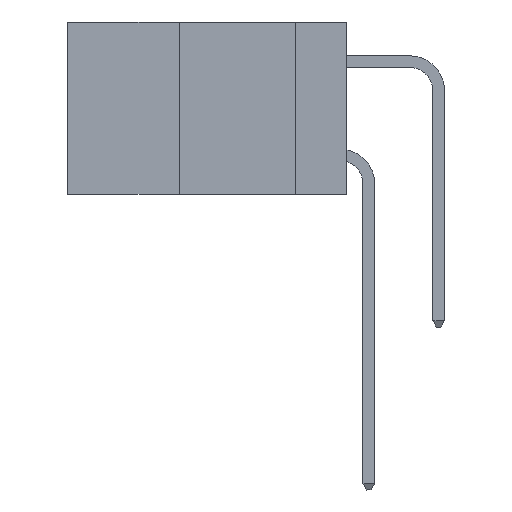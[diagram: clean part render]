
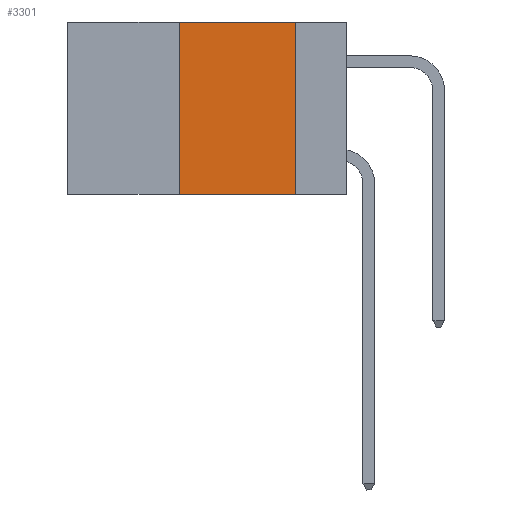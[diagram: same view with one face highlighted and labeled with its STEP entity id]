
A CAD part, left-side view. The second image highlights one B-rep face of the part: STEP entity #3301.
In plain terms, the highlighted planar face has unit normal (-1, 0, 0).
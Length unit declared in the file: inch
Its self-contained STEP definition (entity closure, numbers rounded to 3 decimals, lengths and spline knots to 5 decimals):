
#32 = LINE ( 'NONE', #3934, #11040 ) ;
#1333 = CARTESIAN_POINT ( 'NONE',  ( 0., 0.6, 0. ) ) ;
#1465 = ORIENTED_EDGE ( 'NONE', *, *, #13964, .T. ) ;
#2509 = DIRECTION ( 'NONE',  ( 0., -1., 0. ) ) ;
#3301 = ADVANCED_FACE ( 'NONE', ( #13398 ), #12016, .F. ) ;
#3934 = CARTESIAN_POINT ( 'NONE',  ( 0., 0.36, 0. ) ) ;
#3945 = DIRECTION ( 'NONE',  ( 0., 0., -1. ) ) ;
#3978 = DIRECTION ( 'NONE',  ( 1., 0., 0. ) ) ;
#4523 = EDGE_LOOP ( 'NONE', ( #9824, #4733, #11554, #1465 ) ) ;
#4532 = VECTOR ( 'NONE', #5511, 39.37008 ) ;
#4733 = ORIENTED_EDGE ( 'NONE', *, *, #16162, .F. ) ;
#5443 = CARTESIAN_POINT ( 'NONE',  ( 0., 0.11, 0. ) ) ;
#5511 = DIRECTION ( 'NONE',  ( 0., -1., 0. ) ) ;
#5872 = VERTEX_POINT ( 'NONE', #7890 ) ;
#6411 = LINE ( 'NONE', #7959, #9127 ) ;
#7386 = CARTESIAN_POINT ( 'NONE',  ( 0., 0.36, 0. ) ) ;
#7890 = CARTESIAN_POINT ( 'NONE',  ( 0., 0.11, -0.37 ) ) ;
#7959 = CARTESIAN_POINT ( 'NONE',  ( 0., 0.11, 0. ) ) ;
#7994 = CARTESIAN_POINT ( 'NONE',  ( 0., 0.6, 0. ) ) ;
#8375 = LINE ( 'NONE', #9251, #11103 ) ;
#8546 = CARTESIAN_POINT ( 'NONE',  ( 0., 0.36, -0.37 ) ) ;
#8798 = VERTEX_POINT ( 'NONE', #5443 ) ;
#9127 = VECTOR ( 'NONE', #3945, 39.37008 ) ;
#9251 = CARTESIAN_POINT ( 'NONE',  ( 0., 0.6, -0.37 ) ) ;
#9824 = ORIENTED_EDGE ( 'NONE', *, *, #16711, .F. ) ;
#9827 = VERTEX_POINT ( 'NONE', #8546 ) ;
#11040 = VECTOR ( 'NONE', #14700, 39.37008 ) ;
#11103 = VECTOR ( 'NONE', #2509, 39.37008 ) ;
#11554 = ORIENTED_EDGE ( 'NONE', *, *, #12784, .F. ) ;
#12016 = PLANE ( 'NONE',  #13659 ) ;
#12784 = EDGE_CURVE ( 'NONE', #9827, #15742, #32, .T. ) ;
#13398 = FACE_OUTER_BOUND ( 'NONE', #4523, .T. ) ;
#13431 = DIRECTION ( 'NONE',  ( 0., 0., -1. ) ) ;
#13659 = AXIS2_PLACEMENT_3D ( 'NONE', #7994, #3978, #13431 ) ;
#13964 = EDGE_CURVE ( 'NONE', #9827, #5872, #8375, .T. ) ;
#14700 = DIRECTION ( 'NONE',  ( 0., 0., 1. ) ) ;
#15336 = LINE ( 'NONE', #1333, #4532 ) ;
#15742 = VERTEX_POINT ( 'NONE', #7386 ) ;
#16162 = EDGE_CURVE ( 'NONE', #15742, #8798, #15336, .T. ) ;
#16711 = EDGE_CURVE ( 'NONE', #8798, #5872, #6411, .T. ) ;
